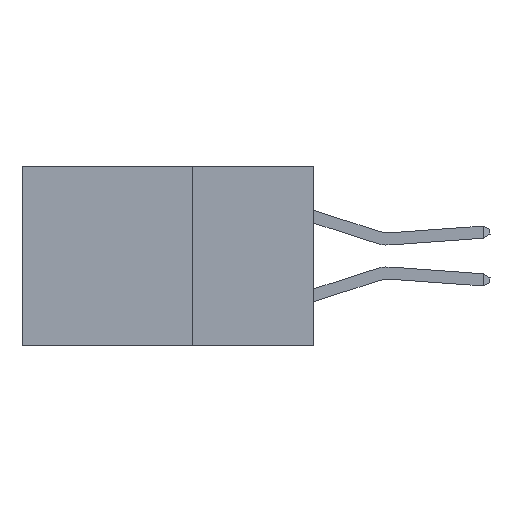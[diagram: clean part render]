
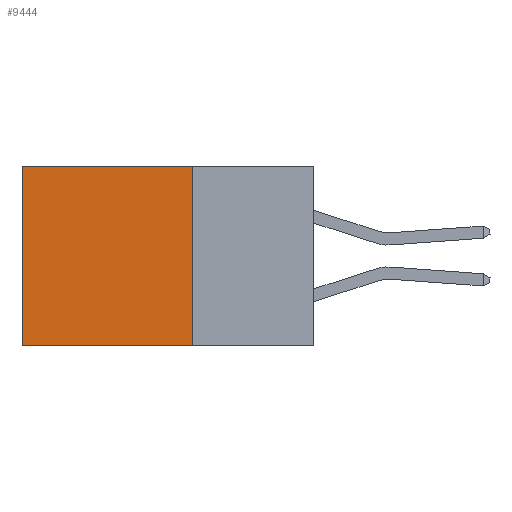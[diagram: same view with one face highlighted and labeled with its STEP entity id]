
A CAD part, left-side view. The second image highlights one B-rep face of the part: STEP entity #9444.
In plain terms, the highlighted planar face has unit normal (-1, 0, 0).
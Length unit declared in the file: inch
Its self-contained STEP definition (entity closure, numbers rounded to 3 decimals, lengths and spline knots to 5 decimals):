
#476 = DIRECTION ( 'NONE',  ( 0., 1., 0. ) ) ;
#491 = ORIENTED_EDGE ( 'NONE', *, *, #8030, .T. ) ;
#1085 = VECTOR ( 'NONE', #2401, 39.37008 ) ;
#1810 = LINE ( 'NONE', #19158, #19302 ) ;
#1865 = LINE ( 'NONE', #17406, #10526 ) ;
#2072 = VERTEX_POINT ( 'NONE', #5330 ) ;
#2401 = DIRECTION ( 'NONE',  ( 0., 1., 0. ) ) ;
#2469 = EDGE_LOOP ( 'NONE', ( #491, #9905, #21951, #6951 ) ) ;
#2693 = VERTEX_POINT ( 'NONE', #8635 ) ;
#5330 = CARTESIAN_POINT ( 'NONE',  ( 0.2875, 0.6, -0.37 ) ) ;
#5685 = DIRECTION ( 'NONE',  ( 0., 0., -1. ) ) ;
#6125 = DIRECTION ( 'NONE',  ( 1., 0., 0. ) ) ;
#6163 = VECTOR ( 'NONE', #10817, 39.37008 ) ;
#6951 = ORIENTED_EDGE ( 'NONE', *, *, #9907, .T. ) ;
#7486 = CARTESIAN_POINT ( 'NONE',  ( 0.2875, 0.25, 0. ) ) ;
#8030 = EDGE_CURVE ( 'NONE', #2693, #2072, #1865, .T. ) ;
#8402 = VERTEX_POINT ( 'NONE', #20143 ) ;
#8635 = CARTESIAN_POINT ( 'NONE',  ( 0.2875, 0.6, 0. ) ) ;
#9444 = ADVANCED_FACE ( 'NONE', ( #19543 ), #21053, .F. ) ;
#9905 = ORIENTED_EDGE ( 'NONE', *, *, #11736, .F. ) ;
#9907 = EDGE_CURVE ( 'NONE', #13463, #2693, #1810, .T. ) ;
#10328 = LINE ( 'NONE', #14346, #1085 ) ;
#10526 = VECTOR ( 'NONE', #5685, 39.37008 ) ;
#10817 = DIRECTION ( 'NONE',  ( 0., 0., -1. ) ) ;
#11736 = EDGE_CURVE ( 'NONE', #8402, #2072, #10328, .T. ) ;
#12360 = AXIS2_PLACEMENT_3D ( 'NONE', #19391, #6125, #17813 ) ;
#13463 = VERTEX_POINT ( 'NONE', #15321 ) ;
#14346 = CARTESIAN_POINT ( 'NONE',  ( 0.2875, 0.25, -0.37 ) ) ;
#15321 = CARTESIAN_POINT ( 'NONE',  ( 0.2875, 0.25, 0. ) ) ;
#17406 = CARTESIAN_POINT ( 'NONE',  ( 0.2875, 0.6, 0. ) ) ;
#17813 = DIRECTION ( 'NONE',  ( 0., 0., -1. ) ) ;
#18948 = LINE ( 'NONE', #7486, #6163 ) ;
#19158 = CARTESIAN_POINT ( 'NONE',  ( 0.2875, 0.25, 0. ) ) ;
#19302 = VECTOR ( 'NONE', #476, 39.37008 ) ;
#19391 = CARTESIAN_POINT ( 'NONE',  ( 0.2875, 0.25, 0. ) ) ;
#19543 = FACE_OUTER_BOUND ( 'NONE', #2469, .T. ) ;
#20143 = CARTESIAN_POINT ( 'NONE',  ( 0.2875, 0.25, -0.37 ) ) ;
#20255 = EDGE_CURVE ( 'NONE', #13463, #8402, #18948, .T. ) ;
#21053 = PLANE ( 'NONE',  #12360 ) ;
#21951 = ORIENTED_EDGE ( 'NONE', *, *, #20255, .F. ) ;
